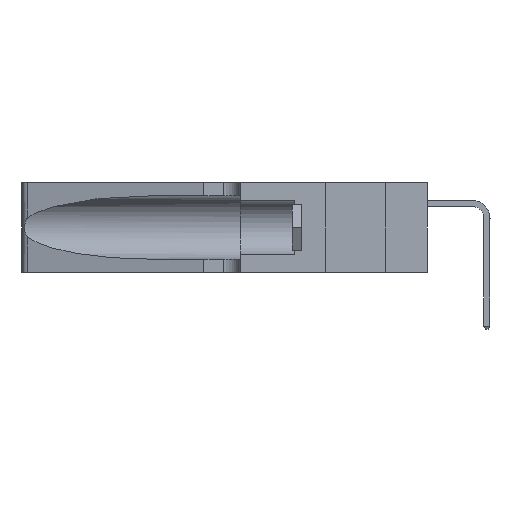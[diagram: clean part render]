
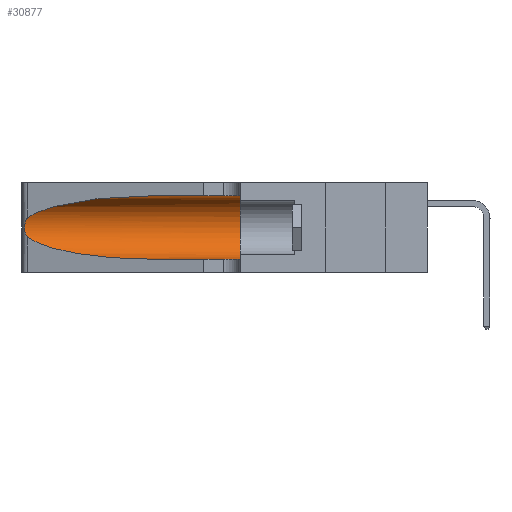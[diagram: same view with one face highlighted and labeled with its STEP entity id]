
A CAD part, left-side view. The second image highlights one B-rep face of the part: STEP entity #30877.
In plain terms, the highlighted cylindrical face has radius 3.308 mm (diameter 6.617 mm), a partial arc.
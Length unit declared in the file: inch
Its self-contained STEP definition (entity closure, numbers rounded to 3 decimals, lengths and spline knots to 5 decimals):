
#24 = CARTESIAN_POINT ( 'NONE',  ( 0.25487, 1.22718, 0.14631 ) ) ;
#93 = DIRECTION ( 'NONE',  ( 0., 0., 1. ) ) ;
#501 = CARTESIAN_POINT ( 'NONE',  ( 0.25487, 1.22718, 0.14631 ) ) ;
#734 = VECTOR ( 'NONE', #3876, 39.37008 ) ;
#744 = EDGE_CURVE ( 'NONE', #17222, #19373, #21146, .T. ) ;
#1317 = CARTESIAN_POINT ( 'NONE',  ( 0.1305, 1.61858, 0.05475 ) ) ;
#1855 =( BOUNDED_CURVE ( )  B_SPLINE_CURVE ( 3, ( #18450, #3563, #20935, #6094 ),
 .UNSPECIFIED., .F., .T. ) 
 B_SPLINE_CURVE_WITH_KNOTS ( ( 4, 4 ),
 ( 1.5708, 2.84003 ),
 .UNSPECIFIED. ) 
 CURVE ( )  GEOMETRIC_REPRESENTATION_ITEM ( )  RATIONAL_B_SPLINE_CURVE ( ( 1., 0.87, 0.87, 1. ) ) 
 REPRESENTATION_ITEM ( '' )  );
#2967 = CARTESIAN_POINT ( 'NONE',  ( 0.25639, 1.23184, 0.21858 ) ) ;
#3449 = VERTEX_POINT ( 'NONE', #12437 ) ;
#3563 = CARTESIAN_POINT ( 'NONE',  ( 0.18966, 0.96281, 0.31525 ) ) ;
#3582 = EDGE_CURVE ( 'NONE', #3449, #17222, #17838, .T. ) ;
#3876 = DIRECTION ( 'NONE',  ( 0., -1., 0. ) ) ;
#5489 = CARTESIAN_POINT ( 'NONE',  ( 0.25854, 1.2359, 0.20912 ) ) ;
#5745 = VERTEX_POINT ( 'NONE', #19458 ) ;
#6094 = CARTESIAN_POINT ( 'NONE',  ( 0.25487, 1.22718, 0.22369 ) ) ;
#7343 = ORIENTED_EDGE ( 'NONE', *, *, #25196, .T. ) ;
#7488 = ORIENTED_EDGE ( 'NONE', *, *, #9098, .T. ) ;
#8011 = LINE ( 'NONE', #30620, #21162 ) ;
#8018 = CARTESIAN_POINT ( 'NONE',  ( 0.26075, 1.23896, 0.19203 ) ) ;
#9098 = EDGE_CURVE ( 'NONE', #19373, #5745, #20639, .T. ) ;
#10032 = ORIENTED_EDGE ( 'NONE', *, *, #14068, .F. ) ;
#10435 = AXIS2_PLACEMENT_3D ( 'NONE', #29849, #15102, #93 ) ;
#10490 = CARTESIAN_POINT ( 'NONE',  ( 0.26017, 1.23833, 0.17102 ) ) ;
#10884 = DIRECTION ( 'NONE',  ( 0., -1., 0. ) ) ;
#11212 = CARTESIAN_POINT ( 'NONE',  ( 0.25487, 1.22718, 0.14631 ) ) ;
#12437 = CARTESIAN_POINT ( 'NONE',  ( 0.25487, 1.22718, 0.22369 ) ) ;
#12984 = CARTESIAN_POINT ( 'NONE',  ( 0.25789, 1.23486, 0.15765 ) ) ;
#13699 = DIRECTION ( 'NONE',  ( 0., 0., -1. ) ) ;
#14068 = EDGE_CURVE ( 'NONE', #27710, #5745, #15325, .T. ) ;
#14264 = AXIS2_PLACEMENT_3D ( 'NONE', #30941, #21151, #13699 ) ;
#14271 = CARTESIAN_POINT ( 'NONE',  ( 0.1305, 0.72297, 0.31525 ) ) ;
#15102 = DIRECTION ( 'NONE',  ( 0., 1., 0. ) ) ;
#15325 = CIRCLE ( 'NONE', #10435, 0.13025 ) ;
#15392 = CARTESIAN_POINT ( 'NONE',  ( 0.25555, 1.22994, 0.2215 ) ) ;
#15454 = EDGE_LOOP ( 'NONE', ( #7343, #18625, #25314, #7488, #10032, #22537 ) ) ;
#15492 = CARTESIAN_POINT ( 'NONE',  ( 0.25555, 1.22993, 0.14849 ) ) ;
#17123 = CARTESIAN_POINT ( 'NONE',  ( 0.1305, 0.72297, 0.05475 ) ) ;
#17222 = VERTEX_POINT ( 'NONE', #11212 ) ;
#17838 = B_SPLINE_CURVE_WITH_KNOTS ( 'NONE', 3,
 ( #25158, #15392, #2967, #20345, #5489, #22815, #8018, #25264, #10490, #27732, #12984, #30228, #15492, #501 ),
 .UNSPECIFIED., .F., .F.,
 ( 4, 2, 2, 2, 2, 2, 4 ),
 ( 0., 0.00027, 0.00053, 0.00107, 0.0016, 0.00187, 0.00214 ),
 .UNSPECIFIED. ) ;
#18450 = CARTESIAN_POINT ( 'NONE',  ( 0.1305, 0.72297, 0.31525 ) ) ;
#18625 = ORIENTED_EDGE ( 'NONE', *, *, #3582, .T. ) ;
#19373 = VERTEX_POINT ( 'NONE', #25121 ) ;
#19458 = CARTESIAN_POINT ( 'NONE',  ( 0.1305, 0.35, 0.05475 ) ) ;
#20345 = CARTESIAN_POINT ( 'NONE',  ( 0.25787, 1.23484, 0.2124 ) ) ;
#20639 = LINE ( 'NONE', #1317, #734 ) ;
#20935 = CARTESIAN_POINT ( 'NONE',  ( 0.2373, 1.15595, 0.28018 ) ) ;
#21146 =( BOUNDED_CURVE ( )  B_SPLINE_CURVE ( 3, ( #24, #22006, #22043, #17123 ),
 .UNSPECIFIED., .F., .F. ) 
 B_SPLINE_CURVE_WITH_KNOTS ( ( 4, 4 ),
 ( 3.44316, 4.71239 ),
 .UNSPECIFIED. ) 
 CURVE ( )  GEOMETRIC_REPRESENTATION_ITEM ( )  RATIONAL_B_SPLINE_CURVE ( ( 1., 0.87, 0.87, 1. ) ) 
 REPRESENTATION_ITEM ( '' )  );
#21151 = DIRECTION ( 'NONE',  ( 0., -1., 0. ) ) ;
#21162 = VECTOR ( 'NONE', #10884, 39.37008 ) ;
#21360 = EDGE_CURVE ( 'NONE', #22027, #27710, #8011, .T. ) ;
#21625 = CARTESIAN_POINT ( 'NONE',  ( 0.1305, 0.35, 0.31525 ) ) ;
#21636 = CYLINDRICAL_SURFACE ( 'NONE', #14264, 0.13025 ) ;
#22006 = CARTESIAN_POINT ( 'NONE',  ( 0.2373, 1.15595, 0.08982 ) ) ;
#22027 = VERTEX_POINT ( 'NONE', #14271 ) ;
#22043 = CARTESIAN_POINT ( 'NONE',  ( 0.18966, 0.96281, 0.05475 ) ) ;
#22537 = ORIENTED_EDGE ( 'NONE', *, *, #21360, .F. ) ;
#22815 = CARTESIAN_POINT ( 'NONE',  ( 0.26018, 1.23835, 0.19895 ) ) ;
#23155 = FACE_OUTER_BOUND ( 'NONE', #15454, .T. ) ;
#25121 = CARTESIAN_POINT ( 'NONE',  ( 0.1305, 0.72297, 0.05475 ) ) ;
#25158 = CARTESIAN_POINT ( 'NONE',  ( 0.25487, 1.22718, 0.22369 ) ) ;
#25196 = EDGE_CURVE ( 'NONE', #22027, #3449, #1855, .T. ) ;
#25264 = CARTESIAN_POINT ( 'NONE',  ( 0.26075, 1.23896, 0.178 ) ) ;
#25314 = ORIENTED_EDGE ( 'NONE', *, *, #744, .T. ) ;
#27710 = VERTEX_POINT ( 'NONE', #21625 ) ;
#27732 = CARTESIAN_POINT ( 'NONE',  ( 0.25856, 1.23593, 0.16098 ) ) ;
#29849 = CARTESIAN_POINT ( 'NONE',  ( 0.1305, 0.35, 0.185 ) ) ;
#30228 = CARTESIAN_POINT ( 'NONE',  ( 0.25639, 1.23186, 0.15144 ) ) ;
#30620 = CARTESIAN_POINT ( 'NONE',  ( 0.1305, 1.61858, 0.31525 ) ) ;
#30877 = ADVANCED_FACE ( 'NONE', ( #23155 ), #21636, .F. ) ;
#30941 = CARTESIAN_POINT ( 'NONE',  ( 0.1305, 1.61858, 0.185 ) ) ;
